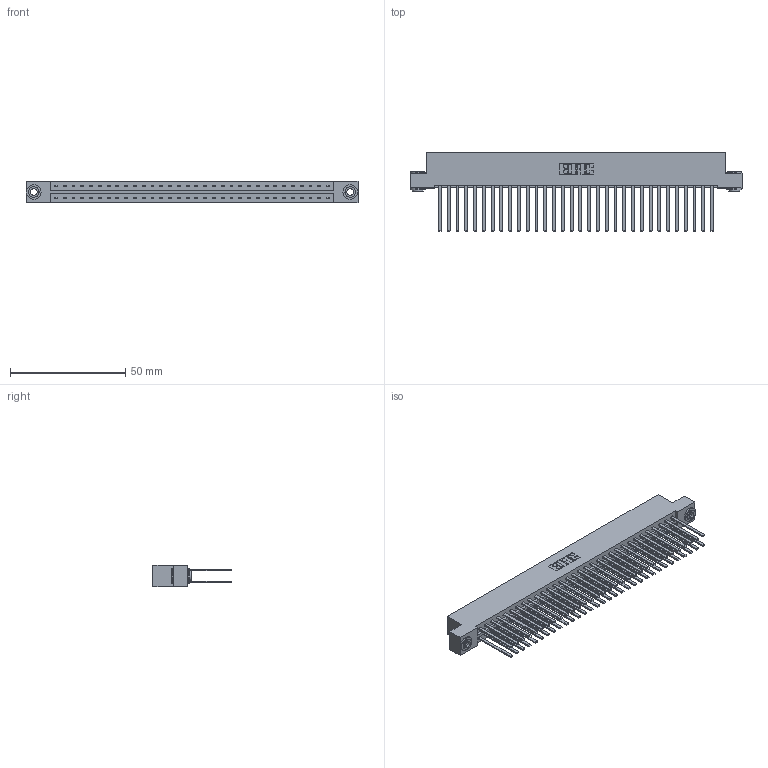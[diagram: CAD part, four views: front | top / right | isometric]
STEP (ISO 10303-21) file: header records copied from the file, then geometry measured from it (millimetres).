
FILE_DESCRIPTION (( 'STEP AP203' ), '1' );
FILE_NAME ('379-064-544-203.STEP', '2020-02-26T18:56:25', ( '' ), ( '' ), 'SwSTEP 2.0', 'SolidWorks 2016', '' );
FILE_SCHEMA (( 'CONFIG_CONTROL_DESIGN' ));
Length unit declared in the file: inch
Products named in the file (4): 379-064-544-203; 379 Part_Flush - .156 Dia - TH; 345-250-002_345-250-002-102; 345-292-001_345-293-144
Assembly tree (67 placements, depth 2):
  379-064-544-203
    379 Part_Flush - .156 Dia - TH
    345-292-001_345-293-144  x64
    345-250-002_345-250-002-102  x2
Bounding box: 144.15 x 33.96 x 9.53 mm (x, y, z)
Volume: 16151.1 mm3; surface area: 21211.3 mm2
Topology: 67 solids, 67 shells, 3096 faces, 9155 edges, 6014 vertices
Faces by surface type: plane 2128, cylinder 960, cone 8
Entity records: 22346 total; most frequent: CARTESIAN_POINT 3689, ORIENTED_EDGE 3618, DIRECTION 3199, EDGE_CURVE 1809, LINE 1661, VECTOR 1661, VERTEX_POINT 1202, AXIS2_PLACEMENT_3D 769
